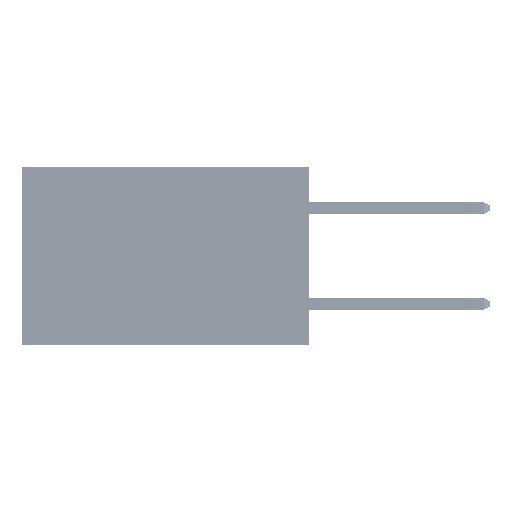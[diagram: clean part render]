
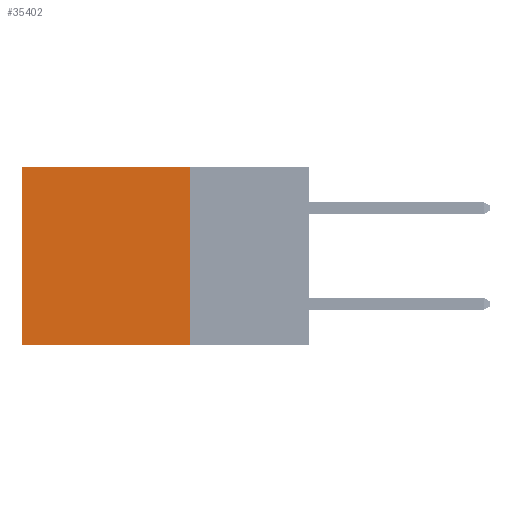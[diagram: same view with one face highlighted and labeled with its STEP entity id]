
A CAD part, left-side view. The second image highlights one B-rep face of the part: STEP entity #35402.
In plain terms, the highlighted planar face has unit normal (-1, 0, 0).
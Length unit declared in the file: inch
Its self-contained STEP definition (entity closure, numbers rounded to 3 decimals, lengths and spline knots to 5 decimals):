
#432 = ORIENTED_EDGE ( 'NONE', *, *, #2419, .T. ) ;
#520 = VERTEX_POINT ( 'NONE', #44456 ) ;
#954 = FACE_OUTER_BOUND ( 'NONE', #41913, .T. ) ;
#1585 = DIRECTION ( 'NONE',  ( 0., 1., 0. ) ) ;
#1837 = EDGE_CURVE ( 'NONE', #36786, #520, #13298, .T. ) ;
#1948 = VERTEX_POINT ( 'NONE', #18814 ) ;
#2419 = EDGE_CURVE ( 'NONE', #520, #1948, #47191, .T. ) ;
#3358 = VECTOR ( 'NONE', #1585, 39.37008 ) ;
#5473 = CARTESIAN_POINT ( 'NONE',  ( 0.2875, 0.25, 0. ) ) ;
#5546 = VECTOR ( 'NONE', #36508, 39.37008 ) ;
#5912 = DIRECTION ( 'NONE',  ( 1., 0., 0. ) ) ;
#9319 = CARTESIAN_POINT ( 'NONE',  ( 0.2875, 0.25, -0.37 ) ) ;
#10526 = ORIENTED_EDGE ( 'NONE', *, *, #24070, .F. ) ;
#11440 = EDGE_CURVE ( 'NONE', #36786, #46674, #21969, .T. ) ;
#11630 = LINE ( 'NONE', #9319, #3358 ) ;
#12110 = CARTESIAN_POINT ( 'NONE',  ( 0.2875, 0.25, 0. ) ) ;
#13298 = LINE ( 'NONE', #47799, #33796 ) ;
#18814 = CARTESIAN_POINT ( 'NONE',  ( 0.2875, 0.6, -0.37 ) ) ;
#20693 = CARTESIAN_POINT ( 'NONE',  ( 0.2875, 0.25, 0. ) ) ;
#21969 = LINE ( 'NONE', #5473, #25473 ) ;
#24070 = EDGE_CURVE ( 'NONE', #46674, #1948, #11630, .T. ) ;
#25370 = DIRECTION ( 'NONE',  ( 0., 1., 0. ) ) ;
#25473 = VECTOR ( 'NONE', #42568, 39.37008 ) ;
#25855 = AXIS2_PLACEMENT_3D ( 'NONE', #20693, #5912, #39072 ) ;
#32065 = CARTESIAN_POINT ( 'NONE',  ( 0.2875, 0.6, 0. ) ) ;
#33796 = VECTOR ( 'NONE', #25370, 39.37008 ) ;
#35402 = ADVANCED_FACE ( 'NONE', ( #954 ), #39242, .F. ) ;
#35620 = ORIENTED_EDGE ( 'NONE', *, *, #11440, .F. ) ;
#36508 = DIRECTION ( 'NONE',  ( 0., 0., -1. ) ) ;
#36786 = VERTEX_POINT ( 'NONE', #12110 ) ;
#39072 = DIRECTION ( 'NONE',  ( 0., 0., -1. ) ) ;
#39242 = PLANE ( 'NONE',  #25855 ) ;
#41035 = CARTESIAN_POINT ( 'NONE',  ( 0.2875, 0.25, -0.37 ) ) ;
#41913 = EDGE_LOOP ( 'NONE', ( #432, #10526, #35620, #46332 ) ) ;
#42568 = DIRECTION ( 'NONE',  ( 0., 0., -1. ) ) ;
#44456 = CARTESIAN_POINT ( 'NONE',  ( 0.2875, 0.6, 0. ) ) ;
#46332 = ORIENTED_EDGE ( 'NONE', *, *, #1837, .T. ) ;
#46674 = VERTEX_POINT ( 'NONE', #41035 ) ;
#47191 = LINE ( 'NONE', #32065, #5546 ) ;
#47799 = CARTESIAN_POINT ( 'NONE',  ( 0.2875, 0.25, 0. ) ) ;
